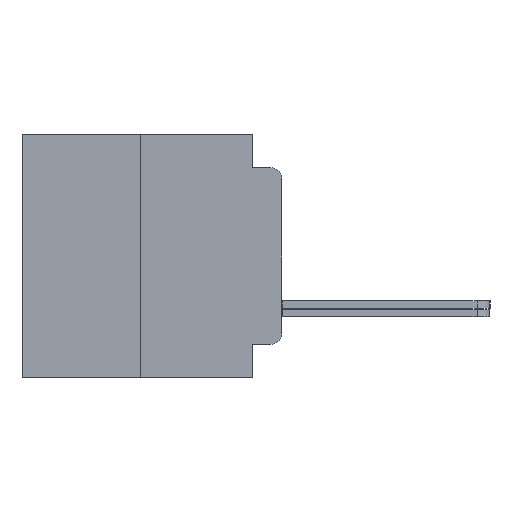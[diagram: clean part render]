
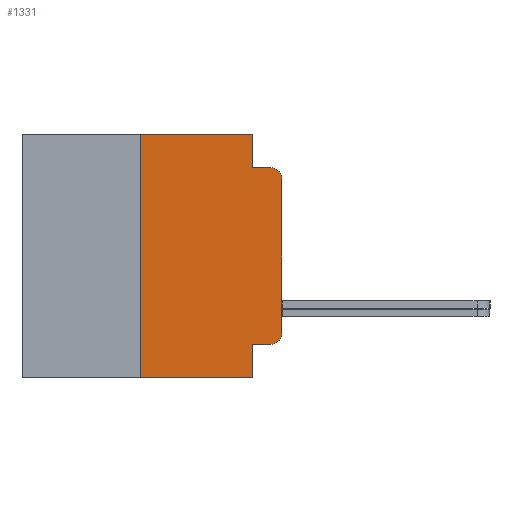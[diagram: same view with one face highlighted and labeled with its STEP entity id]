
A CAD part, left-side view. The second image highlights one B-rep face of the part: STEP entity #1331.
In plain terms, the highlighted planar face has unit normal (-1, 0, 0).
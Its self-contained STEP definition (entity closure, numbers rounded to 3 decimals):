
#98 = DIRECTION ( 'NONE',  ( -1., 0., 0. ) ) ;
#122 = CIRCLE ( 'NONE', #2594, 0.508 ) ;
#649 = CARTESIAN_POINT ( 'NONE',  ( -75.603, 0., 3.467 ) ) ;
#816 = CARTESIAN_POINT ( 'NONE',  ( -75.603, 1.295, -3.975 ) ) ;
#1331 = ADVANCED_FACE ( 'NONE', ( #17434 ), #13364, .F. ) ;
#1374 = DIRECTION ( 'NONE',  ( 0., 0., -1. ) ) ;
#1667 = DIRECTION ( 'NONE',  ( -1., 0., 0. ) ) ;
#1677 = AXIS2_PLACEMENT_3D ( 'NONE', #4302, #19888, #15498 ) ;
#1833 = VECTOR ( 'NONE', #17491, 1000. ) ;
#1934 = CARTESIAN_POINT ( 'NONE',  ( -75.603, 1.295, 3.975 ) ) ;
#1950 = EDGE_CURVE ( 'NONE', #14723, #7652, #20174, .T. ) ;
#2594 = AXIS2_PLACEMENT_3D ( 'NONE', #26750, #98, #15668 ) ;
#3185 = VERTEX_POINT ( 'NONE', #12700 ) ;
#3335 = CARTESIAN_POINT ( 'NONE',  ( -75.603, 1.295, 5.486 ) ) ;
#3789 = DIRECTION ( 'NONE',  ( 0., 0., -1. ) ) ;
#4302 = CARTESIAN_POINT ( 'NONE',  ( -75.603, 11.684, 5.486 ) ) ;
#4471 = LINE ( 'NONE', #23843, #20200 ) ;
#4891 = VECTOR ( 'NONE', #17763, 1000. ) ;
#4894 = VERTEX_POINT ( 'NONE', #9459 ) ;
#5235 = LINE ( 'NONE', #6359, #4891 ) ;
#5639 = ORIENTED_EDGE ( 'NONE', *, *, #25585, .T. ) ;
#6359 = CARTESIAN_POINT ( 'NONE',  ( -75.603, 11.684, 5.486 ) ) ;
#6874 = LINE ( 'NONE', #816, #19073 ) ;
#6949 = VECTOR ( 'NONE', #19420, 1000. ) ;
#7047 = EDGE_CURVE ( 'NONE', #15686, #3185, #25430, .T. ) ;
#7616 = AXIS2_PLACEMENT_3D ( 'NONE', #23656, #1667, #1374 ) ;
#7652 = VERTEX_POINT ( 'NONE', #8807 ) ;
#7798 = ORIENTED_EDGE ( 'NONE', *, *, #16514, .T. ) ;
#8807 = CARTESIAN_POINT ( 'NONE',  ( -75.603, 1.295, 3.975 ) ) ;
#9313 = VERTEX_POINT ( 'NONE', #17209 ) ;
#9459 = CARTESIAN_POINT ( 'NONE',  ( -75.603, 0., -3.467 ) ) ;
#10050 = CARTESIAN_POINT ( 'NONE',  ( -75.603, 0.508, 3.975 ) ) ;
#10553 = ORIENTED_EDGE ( 'NONE', *, *, #7047, .F. ) ;
#10749 = VECTOR ( 'NONE', #3789, 1000. ) ;
#10880 = DIRECTION ( 'NONE',  ( 0., 0., 1. ) ) ;
#10904 = CARTESIAN_POINT ( 'NONE',  ( -75.603, 6.35, -5.486 ) ) ;
#12700 = CARTESIAN_POINT ( 'NONE',  ( -75.603, 1.295, -5.486 ) ) ;
#12889 = VECTOR ( 'NONE', #13131, 1000. ) ;
#13131 = DIRECTION ( 'NONE',  ( 0., 0., -1. ) ) ;
#13364 = PLANE ( 'NONE',  #1677 ) ;
#13581 = LINE ( 'NONE', #23701, #6949 ) ;
#14670 = CARTESIAN_POINT ( 'NONE',  ( -75.603, 6.35, -5.486 ) ) ;
#14723 = VERTEX_POINT ( 'NONE', #3335 ) ;
#15074 = CARTESIAN_POINT ( 'NONE',  ( -75.603, 1.295, 0. ) ) ;
#15175 = CARTESIAN_POINT ( 'NONE',  ( -75.603, 1.295, 0. ) ) ;
#15394 = ORIENTED_EDGE ( 'NONE', *, *, #1950, .F. ) ;
#15498 = DIRECTION ( 'NONE',  ( 0., 0., -1. ) ) ;
#15668 = DIRECTION ( 'NONE',  ( 0., 0., -1. ) ) ;
#15686 = VERTEX_POINT ( 'NONE', #25082 ) ;
#15899 = ORIENTED_EDGE ( 'NONE', *, *, #16561, .T. ) ;
#16514 = EDGE_CURVE ( 'NONE', #15686, #21033, #6874, .T. ) ;
#16554 = ORIENTED_EDGE ( 'NONE', *, *, #22113, .T. ) ;
#16561 = EDGE_CURVE ( 'NONE', #20076, #27730, #18036, .T. ) ;
#17209 = CARTESIAN_POINT ( 'NONE',  ( -75.603, 6.35, 5.486 ) ) ;
#17434 = FACE_OUTER_BOUND ( 'NONE', #28154, .T. ) ;
#17491 = DIRECTION ( 'NONE',  ( 0., -1., 0. ) ) ;
#17763 = DIRECTION ( 'NONE',  ( 0., -1., 0. ) ) ;
#18036 = CIRCLE ( 'NONE', #7616, 0.508 ) ;
#19073 = VECTOR ( 'NONE', #25336, 1000. ) ;
#19260 = DIRECTION ( 'NONE',  ( 0., 0., 1. ) ) ;
#19420 = DIRECTION ( 'NONE',  ( 0., -1., 0. ) ) ;
#19888 = DIRECTION ( 'NONE',  ( 1., 0., 0. ) ) ;
#20076 = VERTEX_POINT ( 'NONE', #649 ) ;
#20174 = LINE ( 'NONE', #15074, #10749 ) ;
#20200 = VECTOR ( 'NONE', #10880, 1000. ) ;
#20493 = CARTESIAN_POINT ( 'NONE',  ( -75.603, 0.508, -3.975 ) ) ;
#20960 = EDGE_CURVE ( 'NONE', #9313, #14723, #5235, .T. ) ;
#21033 = VERTEX_POINT ( 'NONE', #20493 ) ;
#22113 = EDGE_CURVE ( 'NONE', #4894, #20076, #4471, .T. ) ;
#22142 = ORIENTED_EDGE ( 'NONE', *, *, #20960, .F. ) ;
#23422 = ORIENTED_EDGE ( 'NONE', *, *, #26169, .F. ) ;
#23656 = CARTESIAN_POINT ( 'NONE',  ( -75.603, 0.508, 3.467 ) ) ;
#23701 = CARTESIAN_POINT ( 'NONE',  ( -75.603, 11.684, -5.486 ) ) ;
#23843 = CARTESIAN_POINT ( 'NONE',  ( -75.603, 0., 5.486 ) ) ;
#24936 = ORIENTED_EDGE ( 'NONE', *, *, #27304, .T. ) ;
#25082 = CARTESIAN_POINT ( 'NONE',  ( -75.603, 1.295, -3.975 ) ) ;
#25336 = DIRECTION ( 'NONE',  ( 0., -1., 0. ) ) ;
#25430 = LINE ( 'NONE', #15175, #12889 ) ;
#25515 = LINE ( 'NONE', #1934, #1833 ) ;
#25546 = VERTEX_POINT ( 'NONE', #10904 ) ;
#25585 = EDGE_CURVE ( 'NONE', #21033, #4894, #122, .T. ) ;
#25865 = VECTOR ( 'NONE', #19260, 1000. ) ;
#25892 = ORIENTED_EDGE ( 'NONE', *, *, #25941, .F. ) ;
#25941 = EDGE_CURVE ( 'NONE', #25546, #9313, #26561, .T. ) ;
#26169 = EDGE_CURVE ( 'NONE', #7652, #27730, #25515, .T. ) ;
#26561 = LINE ( 'NONE', #14670, #25865 ) ;
#26750 = CARTESIAN_POINT ( 'NONE',  ( -75.603, 0.508, -3.467 ) ) ;
#27304 = EDGE_CURVE ( 'NONE', #25546, #3185, #13581, .T. ) ;
#27730 = VERTEX_POINT ( 'NONE', #10050 ) ;
#28154 = EDGE_LOOP ( 'NONE', ( #7798, #5639, #16554, #15899, #23422, #15394, #22142, #25892, #24936, #10553 ) ) ;
